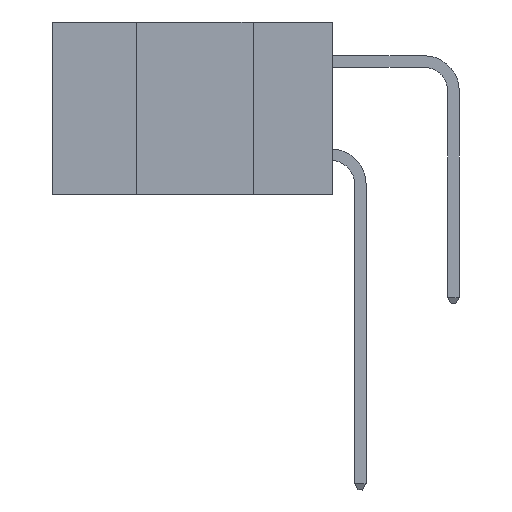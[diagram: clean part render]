
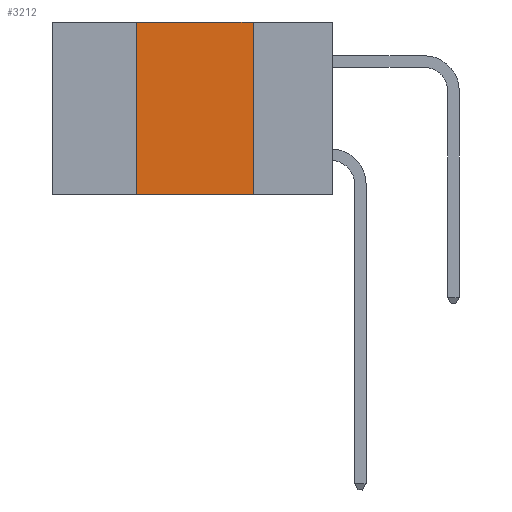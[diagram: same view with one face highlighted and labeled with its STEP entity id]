
A CAD part, left-side view. The second image highlights one B-rep face of the part: STEP entity #3212.
In plain terms, the highlighted planar face has unit normal (-1, 0, 0).
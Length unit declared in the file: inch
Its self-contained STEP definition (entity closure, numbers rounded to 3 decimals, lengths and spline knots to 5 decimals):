
#1758 = VERTEX_POINT ( 'NONE', #15853 ) ;
#2347 = VECTOR ( 'NONE', #3572, 39.37008 ) ;
#2692 = CARTESIAN_POINT ( 'NONE',  ( 0., 0.6, 0. ) ) ;
#2771 = DIRECTION ( 'NONE',  ( 0., 0., 1. ) ) ;
#3025 = VECTOR ( 'NONE', #4447, 39.37008 ) ;
#3212 = ADVANCED_FACE ( 'NONE', ( #18382 ), #16255, .F. ) ;
#3340 = LINE ( 'NONE', #7622, #11522 ) ;
#3572 = DIRECTION ( 'NONE',  ( 0., -1., 0. ) ) ;
#4016 = VERTEX_POINT ( 'NONE', #26094 ) ;
#4447 = DIRECTION ( 'NONE',  ( 0., -1., 0. ) ) ;
#6111 = CARTESIAN_POINT ( 'NONE',  ( 0., 0.6, 0. ) ) ;
#6680 = CARTESIAN_POINT ( 'NONE',  ( 0., 0.42, -0.37 ) ) ;
#7513 = EDGE_CURVE ( 'NONE', #4016, #22688, #10451, .T. ) ;
#7622 = CARTESIAN_POINT ( 'NONE',  ( 0., 0.17, -0.37 ) ) ;
#7726 = LINE ( 'NONE', #19598, #2347 ) ;
#7964 = ORIENTED_EDGE ( 'NONE', *, *, #9913, .T. ) ;
#9722 = CARTESIAN_POINT ( 'NONE',  ( 0., 0.17, -0.37 ) ) ;
#9913 = EDGE_CURVE ( 'NONE', #1758, #16552, #7726, .T. ) ;
#10365 = DIRECTION ( 'NONE',  ( 1., 0., 0. ) ) ;
#10451 = LINE ( 'NONE', #2692, #3025 ) ;
#11522 = VECTOR ( 'NONE', #15764, 39.37008 ) ;
#12766 = ORIENTED_EDGE ( 'NONE', *, *, #16053, .F. ) ;
#15102 = ORIENTED_EDGE ( 'NONE', *, *, #17599, .F. ) ;
#15603 = CARTESIAN_POINT ( 'NONE',  ( 0., 0.17, 0. ) ) ;
#15764 = DIRECTION ( 'NONE',  ( 0., 0., -1. ) ) ;
#15853 = CARTESIAN_POINT ( 'NONE',  ( 0., 0.42, -0.37 ) ) ;
#16053 = EDGE_CURVE ( 'NONE', #22688, #16552, #3340, .T. ) ;
#16174 = AXIS2_PLACEMENT_3D ( 'NONE', #6111, #10365, #24789 ) ;
#16255 = PLANE ( 'NONE',  #16174 ) ;
#16552 = VERTEX_POINT ( 'NONE', #9722 ) ;
#17599 = EDGE_CURVE ( 'NONE', #1758, #4016, #20676, .T. ) ;
#17836 = EDGE_LOOP ( 'NONE', ( #12766, #23661, #15102, #7964 ) ) ;
#18382 = FACE_OUTER_BOUND ( 'NONE', #17836, .T. ) ;
#19598 = CARTESIAN_POINT ( 'NONE',  ( 0., 0.6, -0.37 ) ) ;
#20034 = VECTOR ( 'NONE', #2771, 39.37008 ) ;
#20676 = LINE ( 'NONE', #6680, #20034 ) ;
#22688 = VERTEX_POINT ( 'NONE', #15603 ) ;
#23661 = ORIENTED_EDGE ( 'NONE', *, *, #7513, .F. ) ;
#24789 = DIRECTION ( 'NONE',  ( 0., 0., -1. ) ) ;
#26094 = CARTESIAN_POINT ( 'NONE',  ( 0., 0.42, 0. ) ) ;
